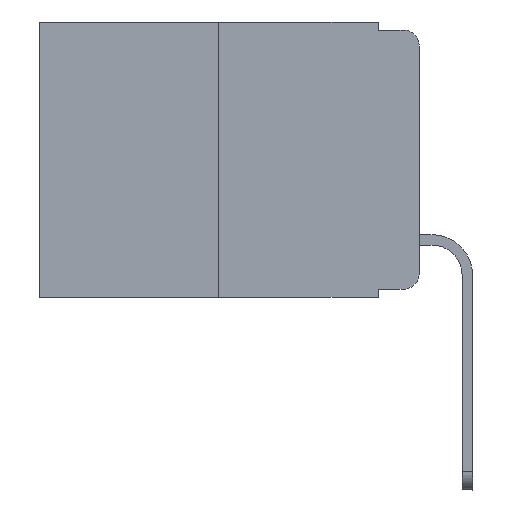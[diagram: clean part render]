
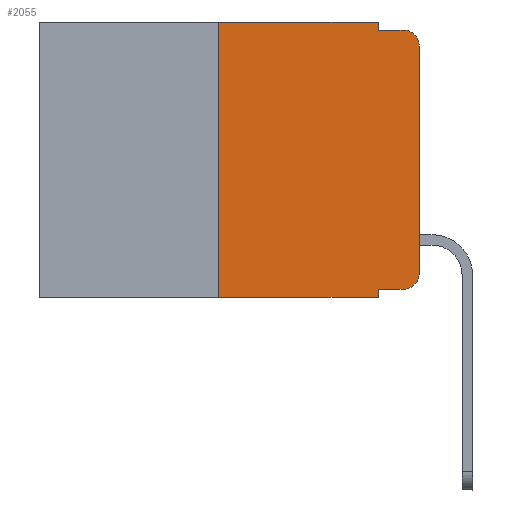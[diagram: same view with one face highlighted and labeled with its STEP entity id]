
A CAD part, left-side view. The second image highlights one B-rep face of the part: STEP entity #2055.
In plain terms, the highlighted planar face has unit normal (-1, 0, 0).
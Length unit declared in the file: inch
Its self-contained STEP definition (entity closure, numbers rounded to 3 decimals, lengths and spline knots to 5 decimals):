
#119 = VERTEX_POINT ( 'NONE', #12051 ) ;
#1053 = DIRECTION ( 'NONE',  ( 0., 0., 1. ) ) ;
#1087 = ORIENTED_EDGE ( 'NONE', *, *, #2682, .T. ) ;
#1143 = CARTESIAN_POINT ( 'NONE',  ( 0., 0.25, 0. ) ) ;
#1650 = VERTEX_POINT ( 'NONE', #11207 ) ;
#1912 = DIRECTION ( 'NONE',  ( 0., 0., 1. ) ) ;
#2055 = ADVANCED_FACE ( 'NONE', ( #18102 ), #5302, .F. ) ;
#2103 = VECTOR ( 'NONE', #1053, 39.37008 ) ;
#2527 = DIRECTION ( 'NONE',  ( 0., -1., 0. ) ) ;
#2660 = DIRECTION ( 'NONE',  ( 0., 0., -1. ) ) ;
#2682 = EDGE_CURVE ( 'NONE', #16851, #3417, #17382, .T. ) ;
#2740 = VECTOR ( 'NONE', #10292, 39.37008 ) ;
#2873 = CARTESIAN_POINT ( 'NONE',  ( 0., 0., -0.313 ) ) ;
#2949 = ORIENTED_EDGE ( 'NONE', *, *, #15187, .F. ) ;
#3413 = ORIENTED_EDGE ( 'NONE', *, *, #5681, .F. ) ;
#3417 = VERTEX_POINT ( 'NONE', #17793 ) ;
#3836 = CARTESIAN_POINT ( 'NONE',  ( 0., 0.02, -0.03 ) ) ;
#4156 = VECTOR ( 'NONE', #8867, 39.37008 ) ;
#4275 = EDGE_CURVE ( 'NONE', #5835, #1650, #8968, .T. ) ;
#4401 = ORIENTED_EDGE ( 'NONE', *, *, #10273, .T. ) ;
#4659 = CARTESIAN_POINT ( 'NONE',  ( 0., 0.473, -0.343 ) ) ;
#4734 = VECTOR ( 'NONE', #1912, 39.37008 ) ;
#4998 = EDGE_CURVE ( 'NONE', #14525, #13097, #7615, .T. ) ;
#5003 = ORIENTED_EDGE ( 'NONE', *, *, #10326, .F. ) ;
#5302 = PLANE ( 'NONE',  #16674 ) ;
#5681 = EDGE_CURVE ( 'NONE', #119, #14123, #10765, .T. ) ;
#5826 = CARTESIAN_POINT ( 'NONE',  ( 0., 0., -0.03 ) ) ;
#5835 = VERTEX_POINT ( 'NONE', #1143 ) ;
#6324 = ORIENTED_EDGE ( 'NONE', *, *, #4275, .F. ) ;
#6377 = CARTESIAN_POINT ( 'NONE',  ( 0., 0.051, 0. ) ) ;
#6383 = ORIENTED_EDGE ( 'NONE', *, *, #13377, .T. ) ;
#7023 = VECTOR ( 'NONE', #12259, 39.37008 ) ;
#7087 = VERTEX_POINT ( 'NONE', #15271 ) ;
#7615 = CIRCLE ( 'NONE', #12363, 0.02 ) ;
#7762 = LINE ( 'NONE', #6377, #14709 ) ;
#7979 = VECTOR ( 'NONE', #9081, 39.37008 ) ;
#8867 = DIRECTION ( 'NONE',  ( 0., -1., 0. ) ) ;
#8931 = ORIENTED_EDGE ( 'NONE', *, *, #10718, .F. ) ;
#8968 = LINE ( 'NONE', #17260, #4156 ) ;
#9081 = DIRECTION ( 'NONE',  ( 0., -1., 0. ) ) ;
#9461 = VECTOR ( 'NONE', #2527, 39.37008 ) ;
#9536 = CARTESIAN_POINT ( 'NONE',  ( 0., 0.051, -0.333 ) ) ;
#9602 = CARTESIAN_POINT ( 'NONE',  ( 0., 0.25, -0.343 ) ) ;
#9702 = CIRCLE ( 'NONE', #14696, 0.02 ) ;
#9894 = ORIENTED_EDGE ( 'NONE', *, *, #14681, .T. ) ;
#10273 = EDGE_CURVE ( 'NONE', #18046, #14123, #9702, .T. ) ;
#10292 = DIRECTION ( 'NONE',  ( 0., -1., 0. ) ) ;
#10326 = EDGE_CURVE ( 'NONE', #7087, #3417, #13617, .T. ) ;
#10718 = EDGE_CURVE ( 'NONE', #1650, #119, #7762, .T. ) ;
#10765 = LINE ( 'NONE', #16106, #7979 ) ;
#11028 = DIRECTION ( 'NONE',  ( 0., 0., -1. ) ) ;
#11207 = CARTESIAN_POINT ( 'NONE',  ( 0., 0.051, 0. ) ) ;
#11253 = DIRECTION ( 'NONE',  ( 0., 0., -1. ) ) ;
#12051 = CARTESIAN_POINT ( 'NONE',  ( 0., 0.051, -0.01 ) ) ;
#12069 = CARTESIAN_POINT ( 'NONE',  ( 0., 0.02, -0.01 ) ) ;
#12259 = DIRECTION ( 'NONE',  ( 0., 0., -1. ) ) ;
#12363 = AXIS2_PLACEMENT_3D ( 'NONE', #13739, #16775, #2660 ) ;
#13097 = VERTEX_POINT ( 'NONE', #2873 ) ;
#13377 = EDGE_CURVE ( 'NONE', #13097, #18046, #13762, .T. ) ;
#13408 = CARTESIAN_POINT ( 'NONE',  ( 0., 0.02, -0.333 ) ) ;
#13617 = LINE ( 'NONE', #16404, #7023 ) ;
#13739 = CARTESIAN_POINT ( 'NONE',  ( 0., 0.02, -0.313 ) ) ;
#13762 = LINE ( 'NONE', #16455, #2103 ) ;
#13774 = CARTESIAN_POINT ( 'NONE',  ( 0., 0.473, 0. ) ) ;
#14123 = VERTEX_POINT ( 'NONE', #12069 ) ;
#14462 = ORIENTED_EDGE ( 'NONE', *, *, #4998, .T. ) ;
#14525 = VERTEX_POINT ( 'NONE', #13408 ) ;
#14681 = EDGE_CURVE ( 'NONE', #7087, #14525, #14897, .T. ) ;
#14696 = AXIS2_PLACEMENT_3D ( 'NONE', #3836, #16492, #15100 ) ;
#14709 = VECTOR ( 'NONE', #11253, 39.37008 ) ;
#14897 = LINE ( 'NONE', #9536, #9461 ) ;
#15100 = DIRECTION ( 'NONE',  ( 0., 0., -1. ) ) ;
#15187 = EDGE_CURVE ( 'NONE', #16851, #5835, #15772, .T. ) ;
#15271 = CARTESIAN_POINT ( 'NONE',  ( 0., 0.051, -0.333 ) ) ;
#15772 = LINE ( 'NONE', #15960, #4734 ) ;
#15960 = CARTESIAN_POINT ( 'NONE',  ( 0., 0.25, 0. ) ) ;
#16106 = CARTESIAN_POINT ( 'NONE',  ( 0., 0.051, -0.01 ) ) ;
#16404 = CARTESIAN_POINT ( 'NONE',  ( 0., 0.051, 0. ) ) ;
#16455 = CARTESIAN_POINT ( 'NONE',  ( 0., 0., 0. ) ) ;
#16492 = DIRECTION ( 'NONE',  ( -1., 0., 0. ) ) ;
#16674 = AXIS2_PLACEMENT_3D ( 'NONE', #13774, #16813, #11028 ) ;
#16775 = DIRECTION ( 'NONE',  ( -1., 0., 0. ) ) ;
#16813 = DIRECTION ( 'NONE',  ( 1., 0., 0. ) ) ;
#16851 = VERTEX_POINT ( 'NONE', #9602 ) ;
#17260 = CARTESIAN_POINT ( 'NONE',  ( 0., 0.473, 0. ) ) ;
#17382 = LINE ( 'NONE', #4659, #2740 ) ;
#17793 = CARTESIAN_POINT ( 'NONE',  ( 0., 0.051, -0.343 ) ) ;
#17862 = EDGE_LOOP ( 'NONE', ( #6383, #4401, #3413, #8931, #6324, #2949, #1087, #5003, #9894, #14462 ) ) ;
#18046 = VERTEX_POINT ( 'NONE', #5826 ) ;
#18102 = FACE_OUTER_BOUND ( 'NONE', #17862, .T. ) ;
